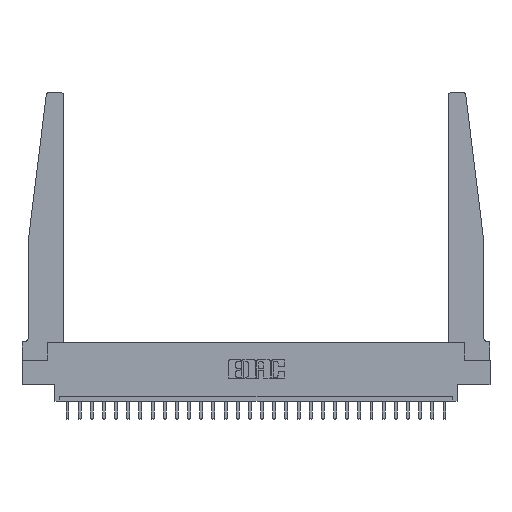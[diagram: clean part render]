
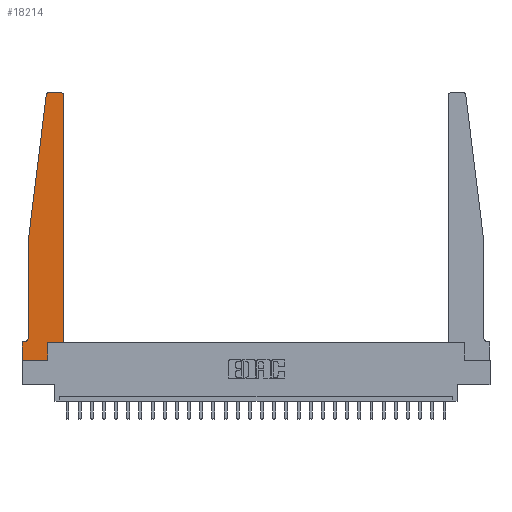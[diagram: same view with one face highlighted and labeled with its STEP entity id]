
A CAD part, top view. The second image highlights one B-rep face of the part: STEP entity #18214.
In plain terms, the highlighted planar face has unit normal (0, 0, 1).
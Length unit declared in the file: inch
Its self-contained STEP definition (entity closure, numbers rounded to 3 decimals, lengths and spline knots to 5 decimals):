
#515 = ORIENTED_EDGE ( 'NONE', *, *, #12780, .T. ) ;
#629 = CARTESIAN_POINT ( 'NONE',  ( 0.015, 0.2375, 0.37 ) ) ;
#871 = EDGE_CURVE ( 'NONE', #8144, #10799, #4935, .T. ) ;
#916 = DIRECTION ( 'NONE',  ( -1., 0., 0. ) ) ;
#1323 = ORIENTED_EDGE ( 'NONE', *, *, #3946, .T. ) ;
#1353 = CARTESIAN_POINT ( 'NONE',  ( 0.065, 1.25, 0.37 ) ) ;
#1404 = CARTESIAN_POINT ( 'NONE',  ( 0.425, 2.72, 0.37 ) ) ;
#1610 = CARTESIAN_POINT ( 'NONE',  ( 0.27653, 2.75, 0.37 ) ) ;
#1683 = EDGE_CURVE ( 'NONE', #2130, #24510, #24806, .T. ) ;
#2130 = VERTEX_POINT ( 'NONE', #3215 ) ;
#2716 = CARTESIAN_POINT ( 'NONE',  ( 0.425, 0.18, 0.37 ) ) ;
#3007 = CARTESIAN_POINT ( 'NONE',  ( 0., 0.1875, 0.37 ) ) ;
#3215 = CARTESIAN_POINT ( 'NONE',  ( 0.425, 0.18, 0.37 ) ) ;
#3224 = DIRECTION ( 'NONE',  ( -0.122, -0.992, 0. ) ) ;
#3293 = EDGE_CURVE ( 'NONE', #6652, #21116, #7324, .T. ) ;
#3709 = EDGE_CURVE ( 'NONE', #10799, #7654, #19298, .T. ) ;
#3759 = DIRECTION ( 'NONE',  ( 1., 0., 0. ) ) ;
#3782 = ORIENTED_EDGE ( 'NONE', *, *, #14656, .T. ) ;
#3946 = EDGE_CURVE ( 'NONE', #24057, #13515, #18354, .T. ) ;
#3954 = ORIENTED_EDGE ( 'NONE', *, *, #10557, .T. ) ;
#4279 = EDGE_CURVE ( 'NONE', #21116, #8144, #22145, .T. ) ;
#4766 = ORIENTED_EDGE ( 'NONE', *, *, #25357, .T. ) ;
#4906 = DIRECTION ( 'NONE',  ( -1., 0., 0. ) ) ;
#4935 = CIRCLE ( 'NONE', #11940, 0.05 ) ;
#5312 = CARTESIAN_POINT ( 'NONE',  ( 0.24675, 2.72367, 0.37 ) ) ;
#5472 = LINE ( 'NONE', #20353, #25695 ) ;
#5982 = ORIENTED_EDGE ( 'NONE', *, *, #4279, .T. ) ;
#6032 = VECTOR ( 'NONE', #11599, 39.37008 ) ;
#6368 = DIRECTION ( 'NONE',  ( 1., 0., 0. ) ) ;
#6652 = VERTEX_POINT ( 'NONE', #5312 ) ;
#7103 = CARTESIAN_POINT ( 'NONE',  ( 0., 0., 0.37 ) ) ;
#7324 = LINE ( 'NONE', #14704, #11398 ) ;
#7529 = CARTESIAN_POINT ( 'NONE',  ( 0.395, 2.75, 0.37 ) ) ;
#7586 = VECTOR ( 'NONE', #21980, 39.37008 ) ;
#7652 = VERTEX_POINT ( 'NONE', #7529 ) ;
#7654 = VERTEX_POINT ( 'NONE', #7778 ) ;
#7778 = CARTESIAN_POINT ( 'NONE',  ( 0., 0.1875, 0.37 ) ) ;
#8144 = VERTEX_POINT ( 'NONE', #19694 ) ;
#8828 = DIRECTION ( 'NONE',  ( 0., -1., 0. ) ) ;
#8913 = CARTESIAN_POINT ( 'NONE',  ( 0., 0., 0.37 ) ) ;
#8925 = EDGE_CURVE ( 'NONE', #7652, #15063, #11530, .T. ) ;
#9847 = CARTESIAN_POINT ( 'NONE',  ( 0.395, 2.72, 0.37 ) ) ;
#10002 = ORIENTED_EDGE ( 'NONE', *, *, #3293, .T. ) ;
#10103 = CARTESIAN_POINT ( 'NONE',  ( 0.2605, 0., 0.37 ) ) ;
#10177 = LINE ( 'NONE', #8913, #10511 ) ;
#10511 = VECTOR ( 'NONE', #8828, 39.37008 ) ;
#10557 = EDGE_CURVE ( 'NONE', #13515, #20016, #5472, .T. ) ;
#10799 = VERTEX_POINT ( 'NONE', #19542 ) ;
#11398 = VECTOR ( 'NONE', #3224, 39.37008 ) ;
#11480 = VECTOR ( 'NONE', #16552, 39.37008 ) ;
#11530 = LINE ( 'NONE', #14477, #20400 ) ;
#11599 = DIRECTION ( 'NONE',  ( 0., -1., 0. ) ) ;
#11940 = AXIS2_PLACEMENT_3D ( 'NONE', #629, #22909, #14755 ) ;
#12097 = AXIS2_PLACEMENT_3D ( 'NONE', #3007, #13232, #19351 ) ;
#12217 = LINE ( 'NONE', #18581, #15395 ) ;
#12378 = EDGE_CURVE ( 'NONE', #15063, #6652, #24016, .T. ) ;
#12780 = EDGE_CURVE ( 'NONE', #24510, #7652, #17034, .T. ) ;
#13232 = DIRECTION ( 'NONE',  ( 0., 0., 1. ) ) ;
#13515 = VERTEX_POINT ( 'NONE', #10103 ) ;
#14119 = ORIENTED_EDGE ( 'NONE', *, *, #3709, .T. ) ;
#14469 = ORIENTED_EDGE ( 'NONE', *, *, #8925, .T. ) ;
#14477 = CARTESIAN_POINT ( 'NONE',  ( 0.25, 2.75, 0.37 ) ) ;
#14656 = EDGE_CURVE ( 'NONE', #7654, #24057, #10177, .T. ) ;
#14704 = CARTESIAN_POINT ( 'NONE',  ( 0.065, 1.25, 0.37 ) ) ;
#14755 = DIRECTION ( 'NONE',  ( -1., 0., 0. ) ) ;
#15063 = VERTEX_POINT ( 'NONE', #1610 ) ;
#15395 = VECTOR ( 'NONE', #6368, 39.37008 ) ;
#15553 = ORIENTED_EDGE ( 'NONE', *, *, #871, .T. ) ;
#15732 = AXIS2_PLACEMENT_3D ( 'NONE', #9847, #15848, #3759 ) ;
#15848 = DIRECTION ( 'NONE',  ( 0., 0., 1. ) ) ;
#16024 = CARTESIAN_POINT ( 'NONE',  ( 0., 0., 0.37 ) ) ;
#16552 = DIRECTION ( 'NONE',  ( 0., 1., 0. ) ) ;
#16771 = DIRECTION ( 'NONE',  ( 1., 0., 0. ) ) ;
#16825 = CARTESIAN_POINT ( 'NONE',  ( 0.065, 0.1875, 0.37 ) ) ;
#17034 = CIRCLE ( 'NONE', #15732, 0.03 ) ;
#18214 = ADVANCED_FACE ( 'NONE', ( #22351 ), #19171, .T. ) ;
#18354 = LINE ( 'NONE', #16024, #7586 ) ;
#18581 = CARTESIAN_POINT ( 'NONE',  ( 0.425, 0.18, 0.37 ) ) ;
#18867 = DIRECTION ( 'NONE',  ( 0., 1., 0. ) ) ;
#19171 = PLANE ( 'NONE',  #12097 ) ;
#19298 = LINE ( 'NONE', #16825, #22453 ) ;
#19351 = DIRECTION ( 'NONE',  ( 1., 0., 0. ) ) ;
#19542 = CARTESIAN_POINT ( 'NONE',  ( 0.015, 0.1875, 0.37 ) ) ;
#19694 = CARTESIAN_POINT ( 'NONE',  ( 0.065, 0.2375, 0.37 ) ) ;
#20016 = VERTEX_POINT ( 'NONE', #20741 ) ;
#20353 = CARTESIAN_POINT ( 'NONE',  ( 0.2605, 0.18, 0.37 ) ) ;
#20400 = VECTOR ( 'NONE', #916, 39.37008 ) ;
#20677 = DIRECTION ( 'NONE',  ( 0., 0., 1. ) ) ;
#20741 = CARTESIAN_POINT ( 'NONE',  ( 0.2605, 0.18, 0.37 ) ) ;
#21116 = VERTEX_POINT ( 'NONE', #25269 ) ;
#21497 = ORIENTED_EDGE ( 'NONE', *, *, #1683, .T. ) ;
#21980 = DIRECTION ( 'NONE',  ( 1., 0., 0. ) ) ;
#22145 = LINE ( 'NONE', #1353, #6032 ) ;
#22351 = FACE_OUTER_BOUND ( 'NONE', #23477, .T. ) ;
#22453 = VECTOR ( 'NONE', #4906, 39.37008 ) ;
#22909 = DIRECTION ( 'NONE',  ( 0., 0., -1. ) ) ;
#23477 = EDGE_LOOP ( 'NONE', ( #14469, #25056, #10002, #5982, #15553, #14119, #3782, #1323, #3954, #4766, #21497, #515 ) ) ;
#23576 = AXIS2_PLACEMENT_3D ( 'NONE', #24940, #20677, #16771 ) ;
#24016 = CIRCLE ( 'NONE', #23576, 0.03 ) ;
#24057 = VERTEX_POINT ( 'NONE', #7103 ) ;
#24510 = VERTEX_POINT ( 'NONE', #1404 ) ;
#24806 = LINE ( 'NONE', #2716, #11480 ) ;
#24940 = CARTESIAN_POINT ( 'NONE',  ( 0.27653, 2.72, 0.37 ) ) ;
#25056 = ORIENTED_EDGE ( 'NONE', *, *, #12378, .T. ) ;
#25269 = CARTESIAN_POINT ( 'NONE',  ( 0.065, 1.25, 0.37 ) ) ;
#25357 = EDGE_CURVE ( 'NONE', #20016, #2130, #12217, .T. ) ;
#25695 = VECTOR ( 'NONE', #18867, 39.37008 ) ;
